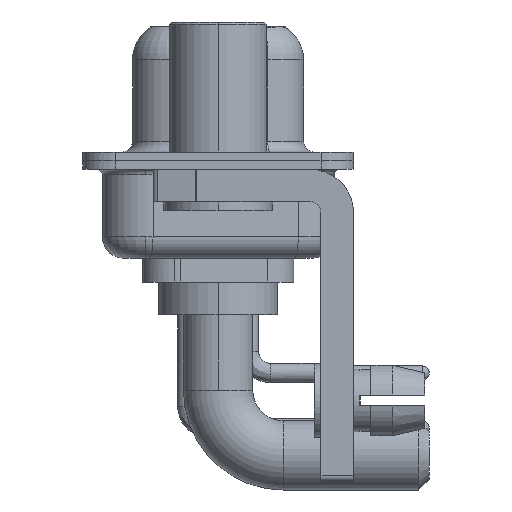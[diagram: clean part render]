
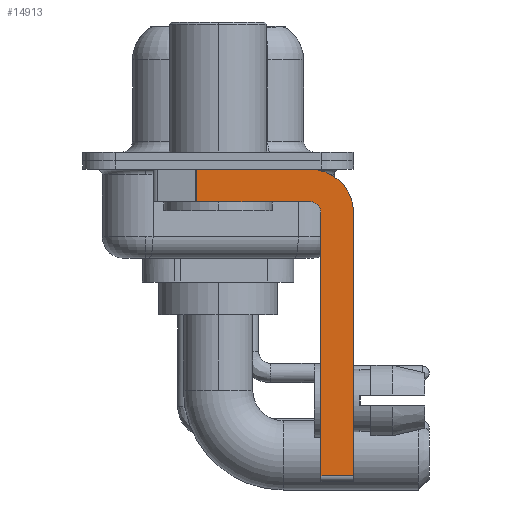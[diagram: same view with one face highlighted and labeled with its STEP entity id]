
A CAD part, left-side view. The second image highlights one B-rep face of the part: STEP entity #14913.
In plain terms, the highlighted planar face has unit normal (-1, 0, 0).
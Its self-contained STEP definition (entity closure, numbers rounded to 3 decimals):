
#422 = CIRCLE ( 'NONE', #5196, 2. ) ;
#620 = CARTESIAN_POINT ( 'NONE',  ( -2.9, -4.25, -2.4 ) ) ;
#1302 = VERTEX_POINT ( 'NONE', #17402 ) ;
#1328 = AXIS2_PLACEMENT_3D ( 'NONE', #22809, #5599, #7802 ) ;
#1417 = CARTESIAN_POINT ( 'NONE',  ( -2.9, 0.978, -1.9 ) ) ;
#1909 = DIRECTION ( 'NONE',  ( 0., 0., -1. ) ) ;
#3121 = CARTESIAN_POINT ( 'NONE',  ( -2.9, 0.978, -1.9 ) ) ;
#3267 = VERTEX_POINT ( 'NONE', #12578 ) ;
#3712 = ORIENTED_EDGE ( 'NONE', *, *, #3916, .F. ) ;
#3916 = EDGE_CURVE ( 'NONE', #3267, #5507, #19272, .T. ) ;
#4318 = CARTESIAN_POINT ( 'NONE',  ( -2.9, 0.978, -0.4 ) ) ;
#5121 = EDGE_CURVE ( 'NONE', #17590, #15205, #422, .T. ) ;
#5196 = AXIS2_PLACEMENT_3D ( 'NONE', #15746, #23232, #13887 ) ;
#5507 = VERTEX_POINT ( 'NONE', #17444 ) ;
#5599 = DIRECTION ( 'NONE',  ( 1., 0., 0. ) ) ;
#5928 = EDGE_CURVE ( 'NONE', #1302, #10800, #10382, .T. ) ;
#6078 = VECTOR ( 'NONE', #23766, 1000. ) ;
#6711 = VERTEX_POINT ( 'NONE', #3121 ) ;
#7802 = DIRECTION ( 'NONE',  ( 0., 0., -1. ) ) ;
#8228 = ORIENTED_EDGE ( 'NONE', *, *, #23719, .T. ) ;
#8596 = CARTESIAN_POINT ( 'NONE',  ( -2.9, -6.25, -14.55 ) ) ;
#8786 = VERTEX_POINT ( 'NONE', #4318 ) ;
#8974 = EDGE_CURVE ( 'NONE', #5507, #6711, #20168, .T. ) ;
#9083 = ORIENTED_EDGE ( 'NONE', *, *, #5928, .T. ) ;
#9106 = VECTOR ( 'NONE', #17414, 1000. ) ;
#9344 = ORIENTED_EDGE ( 'NONE', *, *, #13606, .F. ) ;
#9642 = LINE ( 'NONE', #14840, #12732 ) ;
#9647 = PLANE ( 'NONE',  #1328 ) ;
#10382 = LINE ( 'NONE', #19588, #9106 ) ;
#10800 = VERTEX_POINT ( 'NONE', #8596 ) ;
#11009 = EDGE_LOOP ( 'NONE', ( #16102, #8228, #24265, #3712, #9344, #9083, #16346, #19956 ) ) ;
#11540 = LINE ( 'NONE', #15728, #11649 ) ;
#11649 = VECTOR ( 'NONE', #13631, 1000. ) ;
#11935 = LINE ( 'NONE', #15986, #15236 ) ;
#12297 = DIRECTION ( 'NONE',  ( 0., -1., 0. ) ) ;
#12491 = CARTESIAN_POINT ( 'NONE',  ( -2.9, -6.25, -2.4 ) ) ;
#12578 = CARTESIAN_POINT ( 'NONE',  ( -2.9, -4.75, -2.4 ) ) ;
#12698 = CARTESIAN_POINT ( 'NONE',  ( -2.9, -4.25, -1.9 ) ) ;
#12732 = VECTOR ( 'NONE', #15078, 1000. ) ;
#12800 = EDGE_CURVE ( 'NONE', #8786, #17590, #11935, .T. ) ;
#13013 = AXIS2_PLACEMENT_3D ( 'NONE', #620, #22694, #19358 ) ;
#13117 = FACE_OUTER_BOUND ( 'NONE', #11009, .T. ) ;
#13606 = EDGE_CURVE ( 'NONE', #1302, #3267, #9642, .T. ) ;
#13631 = DIRECTION ( 'NONE',  ( 0., 0., -1. ) ) ;
#13887 = DIRECTION ( 'NONE',  ( 0., 0., -1. ) ) ;
#14840 = CARTESIAN_POINT ( 'NONE',  ( -2.9, -4.75, -14.8 ) ) ;
#14913 = ADVANCED_FACE ( 'NONE', ( #13117 ), #9647, .F. ) ;
#15078 = DIRECTION ( 'NONE',  ( 0., 0., 1. ) ) ;
#15205 = VERTEX_POINT ( 'NONE', #12491 ) ;
#15236 = VECTOR ( 'NONE', #12297, 1000. ) ;
#15728 = CARTESIAN_POINT ( 'NONE',  ( -2.9, -6.25, -2.4 ) ) ;
#15746 = CARTESIAN_POINT ( 'NONE',  ( -2.9, -4.25, -2.4 ) ) ;
#15986 = CARTESIAN_POINT ( 'NONE',  ( -2.9, 3., -0.4 ) ) ;
#16102 = ORIENTED_EDGE ( 'NONE', *, *, #12800, .F. ) ;
#16346 = ORIENTED_EDGE ( 'NONE', *, *, #16460, .F. ) ;
#16460 = EDGE_CURVE ( 'NONE', #15205, #10800, #11540, .T. ) ;
#16700 = CARTESIAN_POINT ( 'NONE',  ( -2.9, -4.25, -0.4 ) ) ;
#16994 = VECTOR ( 'NONE', #1909, 1000. ) ;
#17402 = CARTESIAN_POINT ( 'NONE',  ( -2.9, -4.75, -14.55 ) ) ;
#17414 = DIRECTION ( 'NONE',  ( 0., -1., 0. ) ) ;
#17444 = CARTESIAN_POINT ( 'NONE',  ( -2.9, -4.25, -1.9 ) ) ;
#17590 = VERTEX_POINT ( 'NONE', #16700 ) ;
#18309 = LINE ( 'NONE', #1417, #16994 ) ;
#19272 = CIRCLE ( 'NONE', #13013, 0.5 ) ;
#19358 = DIRECTION ( 'NONE',  ( 0., 0., 1. ) ) ;
#19588 = CARTESIAN_POINT ( 'NONE',  ( -2.9, -4.25, -14.55 ) ) ;
#19956 = ORIENTED_EDGE ( 'NONE', *, *, #5121, .F. ) ;
#20168 = LINE ( 'NONE', #12698, #6078 ) ;
#22694 = DIRECTION ( 'NONE',  ( -1., 0., 0. ) ) ;
#22809 = CARTESIAN_POINT ( 'NONE',  ( -2.9, -4.25, -2.4 ) ) ;
#23232 = DIRECTION ( 'NONE',  ( 1., 0., 0. ) ) ;
#23719 = EDGE_CURVE ( 'NONE', #8786, #6711, #18309, .T. ) ;
#23766 = DIRECTION ( 'NONE',  ( 0., 1., 0. ) ) ;
#24265 = ORIENTED_EDGE ( 'NONE', *, *, #8974, .F. ) ;
